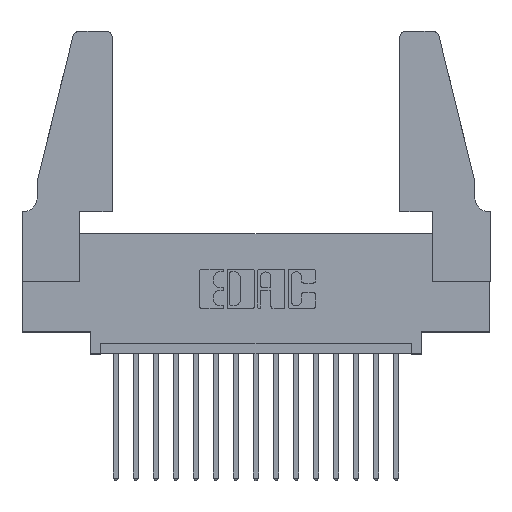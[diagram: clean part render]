
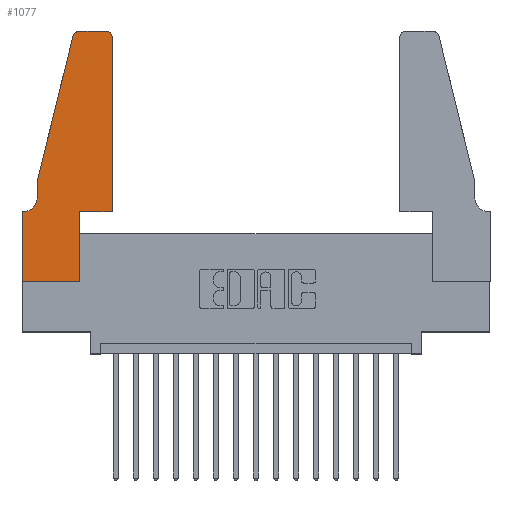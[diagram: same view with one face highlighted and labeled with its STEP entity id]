
A CAD part, top view. The second image highlights one B-rep face of the part: STEP entity #1077.
In plain terms, the highlighted planar face has unit normal (0, 0, 1).
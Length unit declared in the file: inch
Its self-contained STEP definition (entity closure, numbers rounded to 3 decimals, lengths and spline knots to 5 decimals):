
#165 = CARTESIAN_POINT ( 'NONE',  ( 0.4505, 0.35, 0.37 ) ) ;
#238 = DIRECTION ( 'NONE',  ( 1., 0., 0. ) ) ;
#251 = LINE ( 'NONE', #17207, #5042 ) ;
#263 = CARTESIAN_POINT ( 'NONE',  ( 0., 0., 0.37 ) ) ;
#270 = VECTOR ( 'NONE', #8158, 39.37008 ) ;
#288 = CARTESIAN_POINT ( 'NONE',  ( 0.2865, 0.35, 0.37 ) ) ;
#365 = ORIENTED_EDGE ( 'NONE', *, *, #15598, .T. ) ;
#462 = EDGE_CURVE ( 'NONE', #14058, #8185, #16925, .T. ) ;
#811 = EDGE_CURVE ( 'NONE', #7150, #14058, #16910, .T. ) ;
#1077 = ADVANCED_FACE ( 'NONE', ( #4845 ), #2440, .T. ) ;
#1157 = CARTESIAN_POINT ( 'NONE',  ( 0., 0., 0.37 ) ) ;
#1223 = DIRECTION ( 'NONE',  ( 0., 0., 1. ) ) ;
#1574 = CARTESIAN_POINT ( 'NONE',  ( 0.4505, 1.22, 0.37 ) ) ;
#1884 = AXIS2_PLACEMENT_3D ( 'NONE', #13328, #14512, #6628 ) ;
#1941 = ORIENTED_EDGE ( 'NONE', *, *, #7743, .T. ) ;
#2028 = CARTESIAN_POINT ( 'NONE',  ( 0., 0., 0.37 ) ) ;
#2105 = VERTEX_POINT ( 'NONE', #7329 ) ;
#2207 = VERTEX_POINT ( 'NONE', #1574 ) ;
#2440 = PLANE ( 'NONE',  #13411 ) ;
#2754 = LINE ( 'NONE', #165, #13950 ) ;
#3076 = EDGE_CURVE ( 'NONE', #6855, #10975, #251, .T. ) ;
#3189 = EDGE_CURVE ( 'NONE', #2207, #5880, #5988, .T. ) ;
#3327 = CARTESIAN_POINT ( 'NONE',  ( 0., 0.35, 0.37 ) ) ;
#3413 = LINE ( 'NONE', #263, #12942 ) ;
#3454 = VERTEX_POINT ( 'NONE', #12820 ) ;
#3466 = CARTESIAN_POINT ( 'NONE',  ( 0.2865, 0.35, 0.37 ) ) ;
#3629 = DIRECTION ( 'NONE',  ( 0., 0., 1. ) ) ;
#4064 = VECTOR ( 'NONE', #5646, 39.37008 ) ;
#4118 = LINE ( 'NONE', #10827, #14282 ) ;
#4384 = EDGE_CURVE ( 'NONE', #8185, #14504, #3413, .T. ) ;
#4651 = VECTOR ( 'NONE', #5999, 39.37008 ) ;
#4748 = CARTESIAN_POINT ( 'NONE',  ( 0.0055, 0.35, 0.37 ) ) ;
#4845 = FACE_OUTER_BOUND ( 'NONE', #7227, .T. ) ;
#5042 = VECTOR ( 'NONE', #13241, 39.37008 ) ;
#5093 = DIRECTION ( 'NONE',  ( 0., 0., 1. ) ) ;
#5094 = LINE ( 'NONE', #10770, #4064 ) ;
#5189 = ORIENTED_EDGE ( 'NONE', *, *, #462, .T. ) ;
#5203 = ORIENTED_EDGE ( 'NONE', *, *, #6514, .T. ) ;
#5266 = DIRECTION ( 'NONE',  ( 1., 0., 0. ) ) ;
#5646 = DIRECTION ( 'NONE',  ( -1., 0., 0. ) ) ;
#5730 = CARTESIAN_POINT ( 'NONE',  ( 0.284, 1.25, 0.37 ) ) ;
#5802 = CARTESIAN_POINT ( 'NONE',  ( 0.4205, 1.25, 0.37 ) ) ;
#5880 = VERTEX_POINT ( 'NONE', #5802 ) ;
#5988 = CIRCLE ( 'NONE', #16782, 0.03 ) ;
#5999 = DIRECTION ( 'NONE',  ( 0., 1., 0. ) ) ;
#6514 = EDGE_CURVE ( 'NONE', #10975, #3454, #13533, .T. ) ;
#6628 = DIRECTION ( 'NONE',  ( -1., 0., 0. ) ) ;
#6855 = VERTEX_POINT ( 'NONE', #15491 ) ;
#7150 = VERTEX_POINT ( 'NONE', #4748 ) ;
#7162 = CARTESIAN_POINT ( 'NONE',  ( 0.2865, 0., 0.37 ) ) ;
#7225 = CARTESIAN_POINT ( 'NONE',  ( 0.0755, 0.5, 0.37 ) ) ;
#7227 = EDGE_LOOP ( 'NONE', ( #9901, #12310, #12005, #5203, #1941, #12519, #5189, #9687, #8653, #11441, #365, #8669 ) ) ;
#7329 = CARTESIAN_POINT ( 'NONE',  ( 0.4505, 0.35, 0.37 ) ) ;
#7539 = DIRECTION ( 'NONE',  ( 1., 0., 0. ) ) ;
#7743 = EDGE_CURVE ( 'NONE', #3454, #7150, #16826, .T. ) ;
#7895 = CARTESIAN_POINT ( 'NONE',  ( 0.284, 1.22, 0.37 ) ) ;
#8158 = DIRECTION ( 'NONE',  ( -1., 0., 0. ) ) ;
#8185 = VERTEX_POINT ( 'NONE', #2028 ) ;
#8373 = DIRECTION ( 'NONE',  ( 0., 1., 0. ) ) ;
#8653 = ORIENTED_EDGE ( 'NONE', *, *, #16500, .T. ) ;
#8669 = ORIENTED_EDGE ( 'NONE', *, *, #3189, .T. ) ;
#9401 = CIRCLE ( 'NONE', #16581, 0.03 ) ;
#9618 = EDGE_CURVE ( 'NONE', #10857, #6855, #9401, .T. ) ;
#9687 = ORIENTED_EDGE ( 'NONE', *, *, #4384, .T. ) ;
#9882 = CARTESIAN_POINT ( 'NONE',  ( 0.0755, 0.5, 0.37 ) ) ;
#9901 = ORIENTED_EDGE ( 'NONE', *, *, #15856, .T. ) ;
#10770 = CARTESIAN_POINT ( 'NONE',  ( 0.2605, 1.25, 0.37 ) ) ;
#10827 = CARTESIAN_POINT ( 'NONE',  ( 0.4505, 0.35, 0.37 ) ) ;
#10857 = VERTEX_POINT ( 'NONE', #5730 ) ;
#10975 = VERTEX_POINT ( 'NONE', #7225 ) ;
#11423 = CARTESIAN_POINT ( 'NONE',  ( 0.4205, 1.22, 0.37 ) ) ;
#11441 = ORIENTED_EDGE ( 'NONE', *, *, #12175, .T. ) ;
#12001 = DIRECTION ( 'NONE',  ( 0., -1., 0. ) ) ;
#12005 = ORIENTED_EDGE ( 'NONE', *, *, #3076, .T. ) ;
#12175 = EDGE_CURVE ( 'NONE', #16924, #2105, #4118, .T. ) ;
#12310 = ORIENTED_EDGE ( 'NONE', *, *, #9618, .T. ) ;
#12519 = ORIENTED_EDGE ( 'NONE', *, *, #811, .T. ) ;
#12820 = CARTESIAN_POINT ( 'NONE',  ( 0.0755, 0.42, 0.37 ) ) ;
#12942 = VECTOR ( 'NONE', #13696, 39.37008 ) ;
#12943 = CARTESIAN_POINT ( 'NONE',  ( 0., 0.35, 0.37 ) ) ;
#13241 = DIRECTION ( 'NONE',  ( -0.239, -0.971, 0. ) ) ;
#13328 = CARTESIAN_POINT ( 'NONE',  ( 0.0055, 0.42, 0.37 ) ) ;
#13411 = AXIS2_PLACEMENT_3D ( 'NONE', #12943, #5093, #5266 ) ;
#13533 = LINE ( 'NONE', #9882, #14379 ) ;
#13696 = DIRECTION ( 'NONE',  ( 1., 0., 0. ) ) ;
#13807 = VECTOR ( 'NONE', #12001, 39.37008 ) ;
#13950 = VECTOR ( 'NONE', #8373, 39.37008 ) ;
#14054 = DIRECTION ( 'NONE',  ( 0., -1., 0. ) ) ;
#14058 = VERTEX_POINT ( 'NONE', #3327 ) ;
#14282 = VECTOR ( 'NONE', #238, 39.37008 ) ;
#14379 = VECTOR ( 'NONE', #14054, 39.37008 ) ;
#14504 = VERTEX_POINT ( 'NONE', #7162 ) ;
#14512 = DIRECTION ( 'NONE',  ( 0., 0., -1. ) ) ;
#15491 = CARTESIAN_POINT ( 'NONE',  ( 0.25487, 1.22718, 0.37 ) ) ;
#15598 = EDGE_CURVE ( 'NONE', #2105, #2207, #2754, .T. ) ;
#15720 = DIRECTION ( 'NONE',  ( 1., 0., 0. ) ) ;
#15856 = EDGE_CURVE ( 'NONE', #5880, #10857, #5094, .T. ) ;
#16076 = LINE ( 'NONE', #3466, #4651 ) ;
#16123 = CARTESIAN_POINT ( 'NONE',  ( 0.0755, 0.35, 0.37 ) ) ;
#16500 = EDGE_CURVE ( 'NONE', #14504, #16924, #16076, .T. ) ;
#16581 = AXIS2_PLACEMENT_3D ( 'NONE', #7895, #1223, #15720 ) ;
#16782 = AXIS2_PLACEMENT_3D ( 'NONE', #11423, #3629, #7539 ) ;
#16826 = CIRCLE ( 'NONE', #1884, 0.07 ) ;
#16910 = LINE ( 'NONE', #16123, #270 ) ;
#16924 = VERTEX_POINT ( 'NONE', #288 ) ;
#16925 = LINE ( 'NONE', #1157, #13807 ) ;
#17207 = CARTESIAN_POINT ( 'NONE',  ( 0.0755, 0.5, 0.37 ) ) ;
